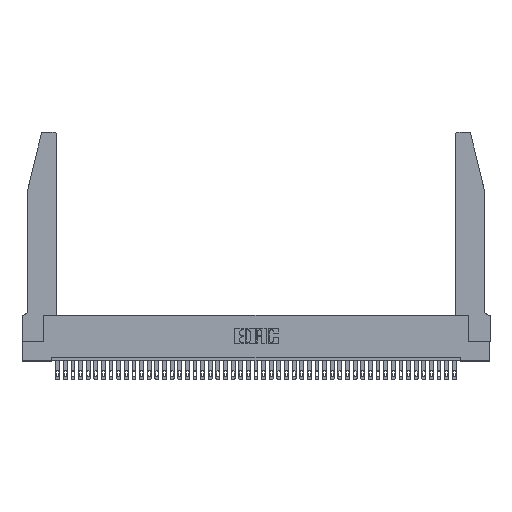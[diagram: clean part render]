
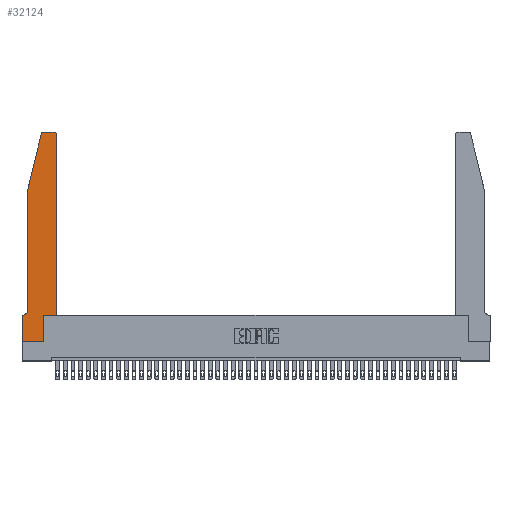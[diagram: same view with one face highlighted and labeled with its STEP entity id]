
A CAD part, top view. The second image highlights one B-rep face of the part: STEP entity #32124.
In plain terms, the highlighted planar face has unit normal (0, 0, 1).
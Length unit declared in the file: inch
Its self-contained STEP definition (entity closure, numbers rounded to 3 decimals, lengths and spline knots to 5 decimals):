
#246 = ORIENTED_EDGE ( 'NONE', *, *, #17703, .T. ) ;
#705 = DIRECTION ( 'NONE',  ( 1., 0., 0. ) ) ;
#1161 = LINE ( 'NONE', #38750, #2702 ) ;
#1277 = VECTOR ( 'NONE', #26917, 39.37008 ) ;
#1915 = CARTESIAN_POINT ( 'NONE',  ( 0.4205, 2.72, 0.37 ) ) ;
#2315 = LINE ( 'NONE', #33623, #23622 ) ;
#2702 = VECTOR ( 'NONE', #5482, 39.37008 ) ;
#3205 = CARTESIAN_POINT ( 'NONE',  ( 0.0755, 2., 0.37 ) ) ;
#4521 = LINE ( 'NONE', #29058, #38843 ) ;
#4880 = CARTESIAN_POINT ( 'NONE',  ( 0.0755, 0.42, 0.37 ) ) ;
#4889 = ORIENTED_EDGE ( 'NONE', *, *, #16182, .T. ) ;
#4914 = CARTESIAN_POINT ( 'NONE',  ( 0.0055, 0.35, 0.37 ) ) ;
#5260 = DIRECTION ( 'NONE',  ( 0., 1., 0. ) ) ;
#5297 = VERTEX_POINT ( 'NONE', #21373 ) ;
#5482 = DIRECTION ( 'NONE',  ( -1., 0., 0. ) ) ;
#5547 = LINE ( 'NONE', #8821, #40931 ) ;
#5943 = ORIENTED_EDGE ( 'NONE', *, *, #42807, .T. ) ;
#6318 = EDGE_CURVE ( 'NONE', #16178, #34834, #2315, .T. ) ;
#7837 = AXIS2_PLACEMENT_3D ( 'NONE', #19531, #39469, #35655 ) ;
#8050 = FACE_OUTER_BOUND ( 'NONE', #26121, .T. ) ;
#8241 = DIRECTION ( 'NONE',  ( 0., -1., 0. ) ) ;
#8549 = EDGE_CURVE ( 'NONE', #18984, #16178, #31768, .T. ) ;
#8821 = CARTESIAN_POINT ( 'NONE',  ( 0., 0., 0.37 ) ) ;
#10594 = CARTESIAN_POINT ( 'NONE',  ( 0.4505, 0.35, 0.37 ) ) ;
#10761 = DIRECTION ( 'NONE',  ( 1., 0., 0. ) ) ;
#12452 = VECTOR ( 'NONE', #15419, 39.37008 ) ;
#13259 = VERTEX_POINT ( 'NONE', #3205 ) ;
#14266 = VERTEX_POINT ( 'NONE', #38569 ) ;
#14907 = VERTEX_POINT ( 'NONE', #28741 ) ;
#15066 = CARTESIAN_POINT ( 'NONE',  ( 0., 0., 0.37 ) ) ;
#15096 = CARTESIAN_POINT ( 'NONE',  ( 0.25487, 2.72718, 0.37 ) ) ;
#15419 = DIRECTION ( 'NONE',  ( 0., 1., 0. ) ) ;
#15800 = AXIS2_PLACEMENT_3D ( 'NONE', #23779, #20453, #705 ) ;
#16178 = VERTEX_POINT ( 'NONE', #23851 ) ;
#16182 = EDGE_CURVE ( 'NONE', #20629, #14266, #38686, .T. ) ;
#16883 = EDGE_CURVE ( 'NONE', #14266, #21368, #17053, .T. ) ;
#16997 = PLANE ( 'NONE',  #15800 ) ;
#17053 = CIRCLE ( 'NONE', #20593, 0.03 ) ;
#17703 = EDGE_CURVE ( 'NONE', #38270, #5297, #5547, .T. ) ;
#17727 = EDGE_CURVE ( 'NONE', #5297, #18984, #27300, .T. ) ;
#17764 = EDGE_CURVE ( 'NONE', #26345, #23963, #26279, .T. ) ;
#18615 = CARTESIAN_POINT ( 'NONE',  ( 0.4205, 2.75, 0.37 ) ) ;
#18750 = CARTESIAN_POINT ( 'NONE',  ( 0.4505, 0.35, 0.37 ) ) ;
#18984 = VERTEX_POINT ( 'NONE', #19608 ) ;
#19001 = ORIENTED_EDGE ( 'NONE', *, *, #16883, .T. ) ;
#19089 = DIRECTION ( 'NONE',  ( -1., 0., 0. ) ) ;
#19531 = CARTESIAN_POINT ( 'NONE',  ( 0.0055, 0.42, 0.37 ) ) ;
#19608 = CARTESIAN_POINT ( 'NONE',  ( 0.2865, 0., 0.37 ) ) ;
#20116 = ORIENTED_EDGE ( 'NONE', *, *, #30718, .T. ) ;
#20269 = CARTESIAN_POINT ( 'NONE',  ( 0.0755, 2., 0.37 ) ) ;
#20453 = DIRECTION ( 'NONE',  ( 0., 0., 1. ) ) ;
#20593 = AXIS2_PLACEMENT_3D ( 'NONE', #37481, #40856, #10761 ) ;
#20629 = VERTEX_POINT ( 'NONE', #18615 ) ;
#20992 = ORIENTED_EDGE ( 'NONE', *, *, #39530, .T. ) ;
#21368 = VERTEX_POINT ( 'NONE', #15096 ) ;
#21373 = CARTESIAN_POINT ( 'NONE',  ( 0., 0., 0.37 ) ) ;
#21971 = ORIENTED_EDGE ( 'NONE', *, *, #8549, .T. ) ;
#22306 = AXIS2_PLACEMENT_3D ( 'NONE', #1915, #35173, #25133 ) ;
#22734 = ORIENTED_EDGE ( 'NONE', *, *, #17764, .T. ) ;
#23059 = VECTOR ( 'NONE', #19089, 39.37008 ) ;
#23622 = VECTOR ( 'NONE', #37125, 39.37008 ) ;
#23779 = CARTESIAN_POINT ( 'NONE',  ( 0., 0.35, 0.37 ) ) ;
#23851 = CARTESIAN_POINT ( 'NONE',  ( 0.2865, 0.35, 0.37 ) ) ;
#23963 = VERTEX_POINT ( 'NONE', #4914 ) ;
#25133 = DIRECTION ( 'NONE',  ( 1., 0., 0. ) ) ;
#25545 = VECTOR ( 'NONE', #5260, 39.37008 ) ;
#25869 = CARTESIAN_POINT ( 'NONE',  ( 0.2605, 2.75, 0.37 ) ) ;
#26121 = EDGE_LOOP ( 'NONE', ( #4889, #19001, #5943, #27367, #22734, #20116, #246, #37544, #21971, #34337, #20992, #32932 ) ) ;
#26279 = CIRCLE ( 'NONE', #7837, 0.07 ) ;
#26345 = VERTEX_POINT ( 'NONE', #4880 ) ;
#26917 = DIRECTION ( 'NONE',  ( -0.239, -0.971, 0. ) ) ;
#27016 = EDGE_CURVE ( 'NONE', #14907, #20629, #28417, .T. ) ;
#27300 = LINE ( 'NONE', #15066, #27809 ) ;
#27367 = ORIENTED_EDGE ( 'NONE', *, *, #27435, .T. ) ;
#27435 = EDGE_CURVE ( 'NONE', #13259, #26345, #4521, .T. ) ;
#27809 = VECTOR ( 'NONE', #28219, 39.37008 ) ;
#28219 = DIRECTION ( 'NONE',  ( 1., 0., 0. ) ) ;
#28417 = CIRCLE ( 'NONE', #22306, 0.03 ) ;
#28741 = CARTESIAN_POINT ( 'NONE',  ( 0.4505, 2.72, 0.37 ) ) ;
#29058 = CARTESIAN_POINT ( 'NONE',  ( 0.0755, 2., 0.37 ) ) ;
#30718 = EDGE_CURVE ( 'NONE', #23963, #38270, #1161, .T. ) ;
#31768 = LINE ( 'NONE', #41767, #25545 ) ;
#32113 = DIRECTION ( 'NONE',  ( 0., -1., 0. ) ) ;
#32124 = ADVANCED_FACE ( 'NONE', ( #8050 ), #16997, .T. ) ;
#32932 = ORIENTED_EDGE ( 'NONE', *, *, #27016, .T. ) ;
#33623 = CARTESIAN_POINT ( 'NONE',  ( 0.4505, 0.35, 0.37 ) ) ;
#34337 = ORIENTED_EDGE ( 'NONE', *, *, #6318, .T. ) ;
#34527 = LINE ( 'NONE', #20269, #1277 ) ;
#34834 = VERTEX_POINT ( 'NONE', #10594 ) ;
#35173 = DIRECTION ( 'NONE',  ( 0., 0., 1. ) ) ;
#35655 = DIRECTION ( 'NONE',  ( -1., 0., 0. ) ) ;
#37125 = DIRECTION ( 'NONE',  ( 1., 0., 0. ) ) ;
#37481 = CARTESIAN_POINT ( 'NONE',  ( 0.284, 2.72, 0.37 ) ) ;
#37544 = ORIENTED_EDGE ( 'NONE', *, *, #17727, .T. ) ;
#37917 = LINE ( 'NONE', #18750, #12452 ) ;
#38270 = VERTEX_POINT ( 'NONE', #41709 ) ;
#38569 = CARTESIAN_POINT ( 'NONE',  ( 0.284, 2.75, 0.37 ) ) ;
#38686 = LINE ( 'NONE', #25869, #23059 ) ;
#38750 = CARTESIAN_POINT ( 'NONE',  ( 0.0755, 0.35, 0.37 ) ) ;
#38843 = VECTOR ( 'NONE', #32113, 39.37008 ) ;
#39469 = DIRECTION ( 'NONE',  ( 0., 0., -1. ) ) ;
#39530 = EDGE_CURVE ( 'NONE', #34834, #14907, #37917, .T. ) ;
#40856 = DIRECTION ( 'NONE',  ( 0., 0., 1. ) ) ;
#40931 = VECTOR ( 'NONE', #8241, 39.37008 ) ;
#41709 = CARTESIAN_POINT ( 'NONE',  ( 0., 0.35, 0.37 ) ) ;
#41767 = CARTESIAN_POINT ( 'NONE',  ( 0.2865, 0.35, 0.37 ) ) ;
#42807 = EDGE_CURVE ( 'NONE', #21368, #13259, #34527, .T. ) ;
